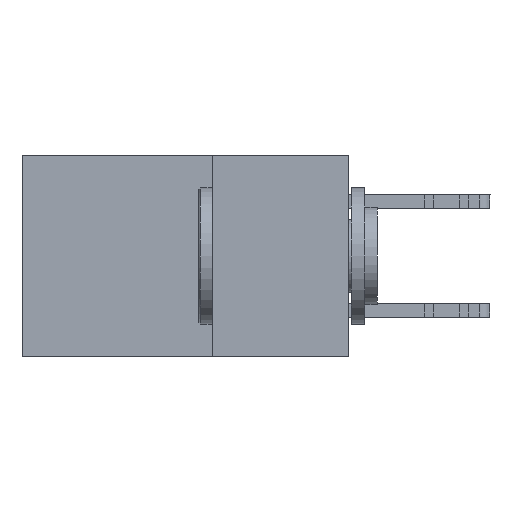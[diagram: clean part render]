
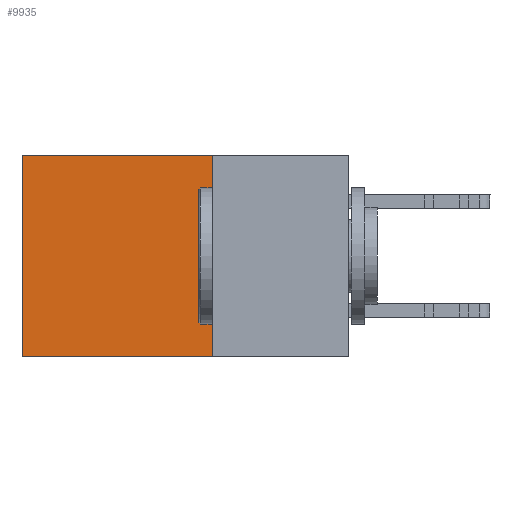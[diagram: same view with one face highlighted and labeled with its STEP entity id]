
A CAD part, left-side view. The second image highlights one B-rep face of the part: STEP entity #9935.
In plain terms, the highlighted planar face has unit normal (-1, 0, 0).
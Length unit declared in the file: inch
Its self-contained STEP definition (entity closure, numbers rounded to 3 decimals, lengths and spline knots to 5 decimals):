
#1533 = VERTEX_POINT ( 'NONE', #12305 ) ;
#1773 = DIRECTION ( 'NONE',  ( 1., 0., 0. ) ) ;
#2423 = CARTESIAN_POINT ( 'NONE',  ( 0.298, 0.25, 0. ) ) ;
#2921 = EDGE_CURVE ( 'NONE', #1533, #13126, #11130, .T. ) ;
#3680 = CARTESIAN_POINT ( 'NONE',  ( 0.298, 0.25, 0. ) ) ;
#4720 = DIRECTION ( 'NONE',  ( 0., 0., -1. ) ) ;
#5705 = DIRECTION ( 'NONE',  ( 0., 0., -1. ) ) ;
#6234 = LINE ( 'NONE', #28029, #10057 ) ;
#6408 = ORIENTED_EDGE ( 'NONE', *, *, #2921, .T. ) ;
#8793 = CARTESIAN_POINT ( 'NONE',  ( 0.298, 0.25, -0.37 ) ) ;
#8961 = CARTESIAN_POINT ( 'NONE',  ( 0.298, 0.6, 0. ) ) ;
#9309 = EDGE_LOOP ( 'NONE', ( #27254, #20625, #18971, #6408 ) ) ;
#9481 = EDGE_CURVE ( 'NONE', #1533, #24046, #16746, .T. ) ;
#9935 = ADVANCED_FACE ( 'NONE', ( #15260 ), #22212, .F. ) ;
#10057 = VECTOR ( 'NONE', #25990, 39.37008 ) ;
#11130 = LINE ( 'NONE', #2423, #19572 ) ;
#11300 = EDGE_CURVE ( 'NONE', #24046, #14735, #6234, .T. ) ;
#12305 = CARTESIAN_POINT ( 'NONE',  ( 0.298, 0.25, 0. ) ) ;
#13126 = VERTEX_POINT ( 'NONE', #8961 ) ;
#13263 = AXIS2_PLACEMENT_3D ( 'NONE', #28482, #1773, #13508 ) ;
#13448 = LINE ( 'NONE', #24758, #20265 ) ;
#13508 = DIRECTION ( 'NONE',  ( 0., 0., -1. ) ) ;
#14735 = VERTEX_POINT ( 'NONE', #26678 ) ;
#15260 = FACE_OUTER_BOUND ( 'NONE', #9309, .T. ) ;
#16494 = DIRECTION ( 'NONE',  ( 0., 1., 0. ) ) ;
#16746 = LINE ( 'NONE', #3680, #18928 ) ;
#17663 = EDGE_CURVE ( 'NONE', #13126, #14735, #13448, .T. ) ;
#18928 = VECTOR ( 'NONE', #5705, 39.37008 ) ;
#18971 = ORIENTED_EDGE ( 'NONE', *, *, #9481, .F. ) ;
#19572 = VECTOR ( 'NONE', #16494, 39.37008 ) ;
#20265 = VECTOR ( 'NONE', #4720, 39.37008 ) ;
#20625 = ORIENTED_EDGE ( 'NONE', *, *, #11300, .F. ) ;
#22212 = PLANE ( 'NONE',  #13263 ) ;
#24046 = VERTEX_POINT ( 'NONE', #8793 ) ;
#24758 = CARTESIAN_POINT ( 'NONE',  ( 0.298, 0.6, 0. ) ) ;
#25990 = DIRECTION ( 'NONE',  ( 0., 1., 0. ) ) ;
#26678 = CARTESIAN_POINT ( 'NONE',  ( 0.298, 0.6, -0.37 ) ) ;
#27254 = ORIENTED_EDGE ( 'NONE', *, *, #17663, .T. ) ;
#28029 = CARTESIAN_POINT ( 'NONE',  ( 0.298, 0.25, -0.37 ) ) ;
#28482 = CARTESIAN_POINT ( 'NONE',  ( 0.298, 0.25, 0. ) ) ;
